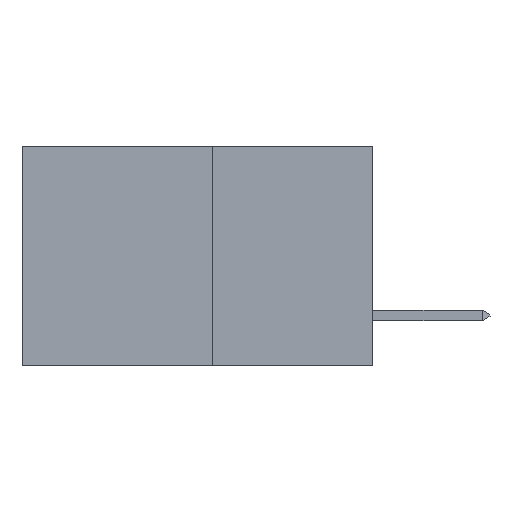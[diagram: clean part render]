
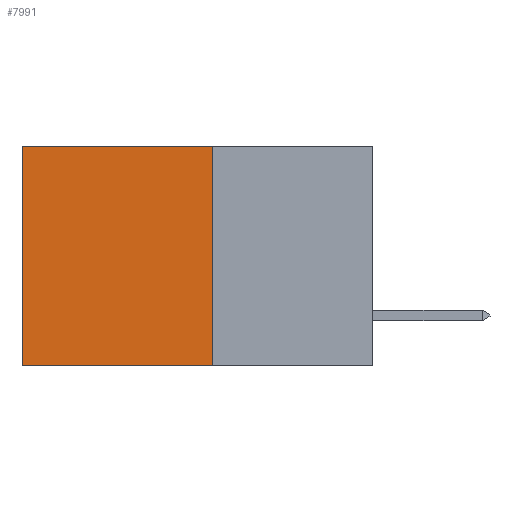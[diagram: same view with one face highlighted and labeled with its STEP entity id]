
A CAD part, left-side view. The second image highlights one B-rep face of the part: STEP entity #7991.
In plain terms, the highlighted planar face has unit normal (-1, 0, 0).
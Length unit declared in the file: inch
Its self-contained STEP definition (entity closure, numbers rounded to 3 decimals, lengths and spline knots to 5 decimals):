
#333 = VERTEX_POINT ( 'NONE', #11602 ) ;
#378 = VECTOR ( 'NONE', #542, 39.37008 ) ;
#542 = DIRECTION ( 'NONE',  ( 0., 0., -1. ) ) ;
#686 = VECTOR ( 'NONE', #5386, 39.37008 ) ;
#777 = CARTESIAN_POINT ( 'NONE',  ( 0.277, 0.27, -0.37 ) ) ;
#833 = VERTEX_POINT ( 'NONE', #11865 ) ;
#887 = ORIENTED_EDGE ( 'NONE', *, *, #2021, .F. ) ;
#957 = ORIENTED_EDGE ( 'NONE', *, *, #1800, .T. ) ;
#1006 = ORIENTED_EDGE ( 'NONE', *, *, #6833, .F. ) ;
#1015 = LINE ( 'NONE', #5223, #686 ) ;
#1473 = ORIENTED_EDGE ( 'NONE', *, *, #3644, .T. ) ;
#1800 = EDGE_CURVE ( 'NONE', #12318, #333, #11774, .T. ) ;
#1835 = VECTOR ( 'NONE', #7822, 39.37008 ) ;
#1889 = CARTESIAN_POINT ( 'NONE',  ( 0.277, 0.59, -0.37 ) ) ;
#2021 = EDGE_CURVE ( 'NONE', #833, #333, #11045, .T. ) ;
#2608 = CARTESIAN_POINT ( 'NONE',  ( 0.277, 0.27, -0.37 ) ) ;
#3488 = EDGE_LOOP ( 'NONE', ( #957, #887, #1006, #1473 ) ) ;
#3636 = DIRECTION ( 'NONE',  ( 1., 0., 0. ) ) ;
#3644 = EDGE_CURVE ( 'NONE', #5077, #12318, #1015, .T. ) ;
#5077 = VERTEX_POINT ( 'NONE', #9034 ) ;
#5223 = CARTESIAN_POINT ( 'NONE',  ( 0.277, 0.27, 0. ) ) ;
#5386 = DIRECTION ( 'NONE',  ( 0., 1., 0. ) ) ;
#6365 = CARTESIAN_POINT ( 'NONE',  ( 0.277, 0.59, 0. ) ) ;
#6600 = AXIS2_PLACEMENT_3D ( 'NONE', #2608, #3636, #10343 ) ;
#6833 = EDGE_CURVE ( 'NONE', #5077, #833, #9342, .T. ) ;
#6955 = DIRECTION ( 'NONE',  ( 0., 1., 0. ) ) ;
#7196 = FACE_OUTER_BOUND ( 'NONE', #3488, .T. ) ;
#7822 = DIRECTION ( 'NONE',  ( 0., 0., -1. ) ) ;
#7991 = ADVANCED_FACE ( 'NONE', ( #7196 ), #8472, .F. ) ;
#8472 = PLANE ( 'NONE',  #6600 ) ;
#9034 = CARTESIAN_POINT ( 'NONE',  ( 0.277, 0.27, 0. ) ) ;
#9342 = LINE ( 'NONE', #777, #1835 ) ;
#10343 = DIRECTION ( 'NONE',  ( 0., 0., -1. ) ) ;
#10753 = VECTOR ( 'NONE', #6955, 39.37008 ) ;
#11045 = LINE ( 'NONE', #11223, #10753 ) ;
#11223 = CARTESIAN_POINT ( 'NONE',  ( 0.277, 0.27, -0.37 ) ) ;
#11602 = CARTESIAN_POINT ( 'NONE',  ( 0.277, 0.59, -0.37 ) ) ;
#11774 = LINE ( 'NONE', #1889, #378 ) ;
#11865 = CARTESIAN_POINT ( 'NONE',  ( 0.277, 0.27, -0.37 ) ) ;
#12318 = VERTEX_POINT ( 'NONE', #6365 ) ;
